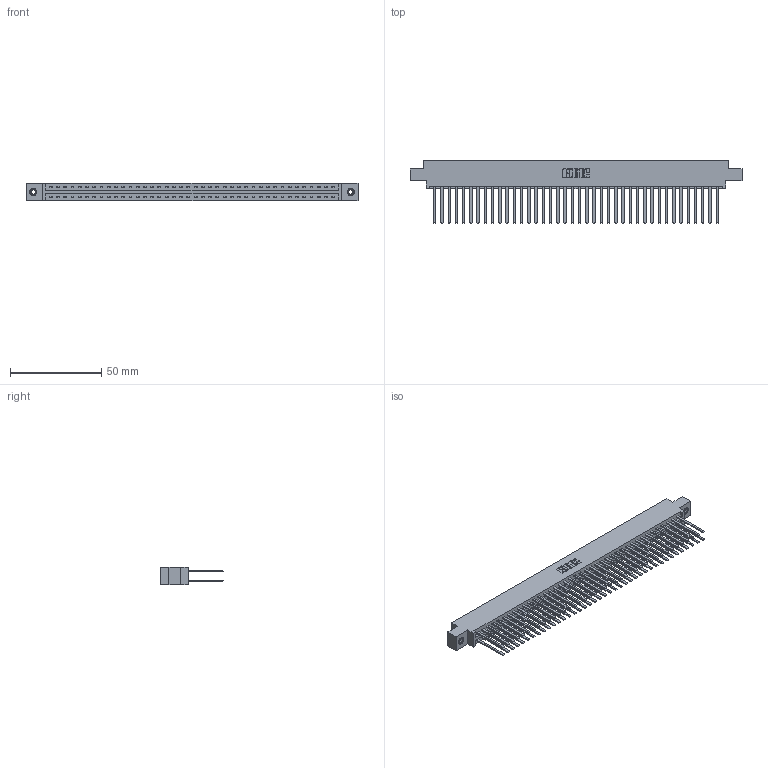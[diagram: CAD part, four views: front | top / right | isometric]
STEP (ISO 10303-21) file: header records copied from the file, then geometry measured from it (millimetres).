
FILE_DESCRIPTION (( 'STEP AP203' ), '1' );
FILE_NAME ('387-080-544-807.STEP', '2019-10-22T22:28:15', ( '' ), ( '' ), 'SwSTEP 2.0', 'SolidWorks 2016', '' );
FILE_SCHEMA (( 'CONFIG_CONTROL_DESIGN' ));
Length unit declared in the file: inch
Products named in the file (4): 345-250-001_345-250-005-103; 345-292-001_345-293-144; 387-080-544-807; 337 Part_0.170 Offset - 0.156 Dia-TI
Assembly tree (83 placements, depth 2):
  387-080-544-807
    337 Part_0.170 Offset - 0.156 Dia-TI
    345-292-001_345-293-144  x80
    345-250-001_345-250-005-103  x2
Bounding box: 181.51 x 34.3 x 9.4 mm (x, y, z)
Volume: 20092.6 mm3; surface area: 26502.6 mm2
Topology: 83 solids, 83 shells, 4018 faces, 11899 edges, 7818 vertices
Faces by surface type: plane 2826, cylinder 1176, cone 12, torus 4
Entity records: 32406 total; most frequent: CARTESIAN_POINT 5441, ORIENTED_EDGE 5370, DIRECTION 4659, EDGE_CURVE 2685, LINE 2541, VECTOR 2541, VERTEX_POINT 1784, AXIS2_PLACEMENT_3D 1059
